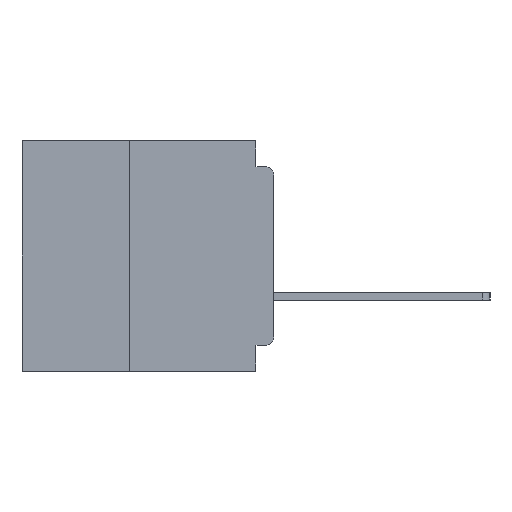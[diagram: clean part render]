
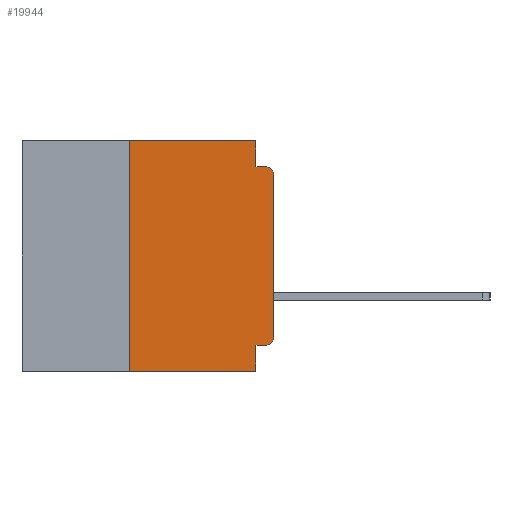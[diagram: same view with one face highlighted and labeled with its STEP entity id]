
A CAD part, left-side view. The second image highlights one B-rep face of the part: STEP entity #19944.
In plain terms, the highlighted planar face has unit normal (-1, 0, 0).
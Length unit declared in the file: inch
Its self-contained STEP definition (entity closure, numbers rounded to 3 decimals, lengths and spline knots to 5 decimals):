
#105 = DIRECTION ( 'NONE',  ( 0., 0., -1. ) ) ;
#151 = VERTEX_POINT ( 'NONE', #3832 ) ;
#1506 = FACE_OUTER_BOUND ( 'NONE', #37296, .T. ) ;
#2270 = EDGE_CURVE ( 'NONE', #37173, #151, #27703, .T. ) ;
#2826 = DIRECTION ( 'NONE',  ( 0., -1., 0. ) ) ;
#3061 = DIRECTION ( 'NONE',  ( 0., 0., -1. ) ) ;
#3832 = CARTESIAN_POINT ( 'NONE',  ( 0., 0.031, -0.4 ) ) ;
#4300 = ORIENTED_EDGE ( 'NONE', *, *, #37032, .T. ) ;
#4856 = VERTEX_POINT ( 'NONE', #34643 ) ;
#5048 = VERTEX_POINT ( 'NONE', #7231 ) ;
#6069 = DIRECTION ( 'NONE',  ( 0., 0., -1. ) ) ;
#6234 = VECTOR ( 'NONE', #41127, 39.37008 ) ;
#7231 = CARTESIAN_POINT ( 'NONE',  ( 0., 0.031, 0. ) ) ;
#7970 = AXIS2_PLACEMENT_3D ( 'NONE', #38127, #19269, #105 ) ;
#8292 = CARTESIAN_POINT ( 'NONE',  ( 0., 0.25, -0.4 ) ) ;
#8370 = DIRECTION ( 'NONE',  ( 0., 1., 0. ) ) ;
#8531 = CARTESIAN_POINT ( 'NONE',  ( 0., 0., -0.34 ) ) ;
#9855 = CARTESIAN_POINT ( 'NONE',  ( 0., 0.437, 0. ) ) ;
#10091 = VERTEX_POINT ( 'NONE', #39375 ) ;
#10763 = EDGE_CURVE ( 'NONE', #21264, #5048, #37548, .T. ) ;
#10812 = VECTOR ( 'NONE', #37142, 39.37008 ) ;
#11358 = VECTOR ( 'NONE', #23766, 39.37008 ) ;
#11850 = LINE ( 'NONE', #8292, #19333 ) ;
#12015 = VERTEX_POINT ( 'NONE', #8531 ) ;
#12204 = EDGE_CURVE ( 'NONE', #4856, #23092, #31552, .T. ) ;
#13075 = DIRECTION ( 'NONE',  ( 1., 0., 0. ) ) ;
#13678 = AXIS2_PLACEMENT_3D ( 'NONE', #9855, #13075, #35168 ) ;
#15140 = CARTESIAN_POINT ( 'NONE',  ( 0., 0.031, -0.355 ) ) ;
#17533 = EDGE_CURVE ( 'NONE', #31976, #12015, #39906, .T. ) ;
#18243 = VECTOR ( 'NONE', #8370, 39.37008 ) ;
#18497 = ORIENTED_EDGE ( 'NONE', *, *, #12204, .F. ) ;
#18855 = VECTOR ( 'NONE', #6069, 39.37008 ) ;
#19269 = DIRECTION ( 'NONE',  ( -1., 0., 0. ) ) ;
#19333 = VECTOR ( 'NONE', #27168, 39.37008 ) ;
#19565 = ORIENTED_EDGE ( 'NONE', *, *, #17533, .T. ) ;
#19874 = LINE ( 'NONE', #28168, #18855 ) ;
#19944 = ADVANCED_FACE ( 'NONE', ( #1506 ), #28853, .F. ) ;
#20262 = LINE ( 'NONE', #24212, #18243 ) ;
#21131 = AXIS2_PLACEMENT_3D ( 'NONE', #41041, #22224, #3061 ) ;
#21264 = VERTEX_POINT ( 'NONE', #39710 ) ;
#22224 = DIRECTION ( 'NONE',  ( -1., 0., 0. ) ) ;
#22226 = LINE ( 'NONE', #33358, #37952 ) ;
#23092 = VERTEX_POINT ( 'NONE', #40278 ) ;
#23766 = DIRECTION ( 'NONE',  ( 0., -1., 0. ) ) ;
#24051 = VERTEX_POINT ( 'NONE', #40325 ) ;
#24212 = CARTESIAN_POINT ( 'NONE',  ( 0., 0., -0.355 ) ) ;
#25570 = ORIENTED_EDGE ( 'NONE', *, *, #10763, .F. ) ;
#25870 = ORIENTED_EDGE ( 'NONE', *, *, #2270, .F. ) ;
#26002 = EDGE_CURVE ( 'NONE', #10091, #151, #29287, .T. ) ;
#26520 = EDGE_CURVE ( 'NONE', #5048, #4856, #19874, .T. ) ;
#27168 = DIRECTION ( 'NONE',  ( 0., 0., 1. ) ) ;
#27602 = EDGE_CURVE ( 'NONE', #31976, #37173, #20262, .T. ) ;
#27703 = LINE ( 'NONE', #37551, #10812 ) ;
#28168 = CARTESIAN_POINT ( 'NONE',  ( 0., 0.031, 0. ) ) ;
#28320 = CARTESIAN_POINT ( 'NONE',  ( 0., 0.437, -0.4 ) ) ;
#28717 = EDGE_CURVE ( 'NONE', #10091, #21264, #11850, .T. ) ;
#28853 = PLANE ( 'NONE',  #13678 ) ;
#29287 = LINE ( 'NONE', #28320, #37616 ) ;
#29729 = ORIENTED_EDGE ( 'NONE', *, *, #26520, .F. ) ;
#30320 = ORIENTED_EDGE ( 'NONE', *, *, #28717, .F. ) ;
#31552 = LINE ( 'NONE', #37970, #6234 ) ;
#31756 = CARTESIAN_POINT ( 'NONE',  ( 0., 0.015, -0.355 ) ) ;
#31976 = VERTEX_POINT ( 'NONE', #31756 ) ;
#33248 = CARTESIAN_POINT ( 'NONE',  ( 0., 0.437, 0. ) ) ;
#33358 = CARTESIAN_POINT ( 'NONE',  ( 0., 0., 0. ) ) ;
#34643 = CARTESIAN_POINT ( 'NONE',  ( 0., 0.031, -0.045 ) ) ;
#35150 = EDGE_CURVE ( 'NONE', #24051, #23092, #39610, .T. ) ;
#35168 = DIRECTION ( 'NONE',  ( 0., 0., -1. ) ) ;
#35527 = ORIENTED_EDGE ( 'NONE', *, *, #35150, .T. ) ;
#36212 = ORIENTED_EDGE ( 'NONE', *, *, #27602, .F. ) ;
#36509 = DIRECTION ( 'NONE',  ( 0., 0., 1. ) ) ;
#36899 = ORIENTED_EDGE ( 'NONE', *, *, #26002, .T. ) ;
#37032 = EDGE_CURVE ( 'NONE', #12015, #24051, #22226, .T. ) ;
#37142 = DIRECTION ( 'NONE',  ( 0., 0., -1. ) ) ;
#37173 = VERTEX_POINT ( 'NONE', #15140 ) ;
#37296 = EDGE_LOOP ( 'NONE', ( #4300, #35527, #18497, #29729, #25570, #30320, #36899, #25870, #36212, #19565 ) ) ;
#37548 = LINE ( 'NONE', #33248, #11358 ) ;
#37551 = CARTESIAN_POINT ( 'NONE',  ( 0., 0.031, -0.4 ) ) ;
#37616 = VECTOR ( 'NONE', #2826, 39.37008 ) ;
#37952 = VECTOR ( 'NONE', #36509, 39.37008 ) ;
#37970 = CARTESIAN_POINT ( 'NONE',  ( 0., 0., -0.045 ) ) ;
#38127 = CARTESIAN_POINT ( 'NONE',  ( 0., 0.015, -0.34 ) ) ;
#39375 = CARTESIAN_POINT ( 'NONE',  ( 0., 0.25, -0.4 ) ) ;
#39610 = CIRCLE ( 'NONE', #21131, 0.015 ) ;
#39710 = CARTESIAN_POINT ( 'NONE',  ( 0., 0.25, 0. ) ) ;
#39906 = CIRCLE ( 'NONE', #7970, 0.015 ) ;
#40278 = CARTESIAN_POINT ( 'NONE',  ( 0., 0.015, -0.045 ) ) ;
#40325 = CARTESIAN_POINT ( 'NONE',  ( 0., 0., -0.06 ) ) ;
#41041 = CARTESIAN_POINT ( 'NONE',  ( 0., 0.015, -0.06 ) ) ;
#41127 = DIRECTION ( 'NONE',  ( 0., -1., 0. ) ) ;
